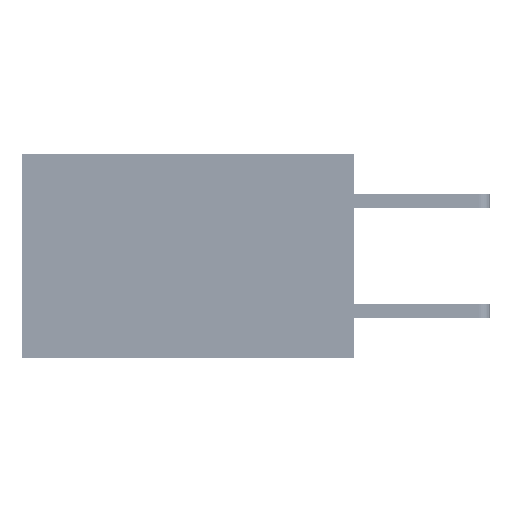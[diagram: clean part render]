
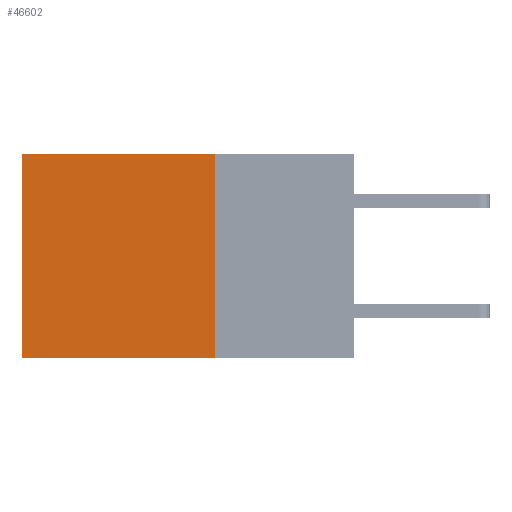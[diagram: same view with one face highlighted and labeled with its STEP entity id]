
A CAD part, left-side view. The second image highlights one B-rep face of the part: STEP entity #46602.
In plain terms, the highlighted planar face has unit normal (-1, 0, 0).
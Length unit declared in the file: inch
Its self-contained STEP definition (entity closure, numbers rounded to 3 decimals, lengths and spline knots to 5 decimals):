
#493 = VERTEX_POINT ( 'NONE', #17430 ) ;
#2474 = EDGE_CURVE ( 'NONE', #16508, #493, #9214, .T. ) ;
#2697 = EDGE_CURVE ( 'NONE', #493, #24731, #45174, .T. ) ;
#6767 = DIRECTION ( 'NONE',  ( 0., 1., 0. ) ) ;
#7314 = VERTEX_POINT ( 'NONE', #22555 ) ;
#7531 = LINE ( 'NONE', #25855, #24650 ) ;
#9214 = LINE ( 'NONE', #24003, #32315 ) ;
#10503 = CARTESIAN_POINT ( 'NONE',  ( 0.2875, 0.25, 0. ) ) ;
#10666 = PLANE ( 'NONE',  #19569 ) ;
#11275 = DIRECTION ( 'NONE',  ( 0., 1., 0. ) ) ;
#12740 = CARTESIAN_POINT ( 'NONE',  ( 0.2875, 0.25, 0. ) ) ;
#13717 = LINE ( 'NONE', #43573, #48816 ) ;
#15975 = ORIENTED_EDGE ( 'NONE', *, *, #18605, .T. ) ;
#16197 = EDGE_CURVE ( 'NONE', #16508, #7314, #7531, .T. ) ;
#16508 = VERTEX_POINT ( 'NONE', #12740 ) ;
#17430 = CARTESIAN_POINT ( 'NONE',  ( 0.2875, 0.25, -0.37 ) ) ;
#18501 = CARTESIAN_POINT ( 'NONE',  ( 0.2875, 0.25, -0.37 ) ) ;
#18605 = EDGE_CURVE ( 'NONE', #7314, #24731, #13717, .T. ) ;
#19569 = AXIS2_PLACEMENT_3D ( 'NONE', #10503, #37025, #29389 ) ;
#19674 = ORIENTED_EDGE ( 'NONE', *, *, #16197, .T. ) ;
#22555 = CARTESIAN_POINT ( 'NONE',  ( 0.2875, 0.6, 0. ) ) ;
#24003 = CARTESIAN_POINT ( 'NONE',  ( 0.2875, 0.25, 0. ) ) ;
#24650 = VECTOR ( 'NONE', #11275, 39.37008 ) ;
#24731 = VERTEX_POINT ( 'NONE', #42796 ) ;
#25855 = CARTESIAN_POINT ( 'NONE',  ( 0.2875, 0.25, 0. ) ) ;
#27207 = DIRECTION ( 'NONE',  ( 0., 0., -1. ) ) ;
#29389 = DIRECTION ( 'NONE',  ( 0., 0., -1. ) ) ;
#32315 = VECTOR ( 'NONE', #27207, 39.37008 ) ;
#37025 = DIRECTION ( 'NONE',  ( 1., 0., 0. ) ) ;
#37206 = ORIENTED_EDGE ( 'NONE', *, *, #2697, .F. ) ;
#37350 = FACE_OUTER_BOUND ( 'NONE', #39939, .T. ) ;
#39799 = VECTOR ( 'NONE', #6767, 39.37008 ) ;
#39939 = EDGE_LOOP ( 'NONE', ( #15975, #37206, #40849, #19674 ) ) ;
#40849 = ORIENTED_EDGE ( 'NONE', *, *, #2474, .F. ) ;
#42796 = CARTESIAN_POINT ( 'NONE',  ( 0.2875, 0.6, -0.37 ) ) ;
#43418 = DIRECTION ( 'NONE',  ( 0., 0., -1. ) ) ;
#43573 = CARTESIAN_POINT ( 'NONE',  ( 0.2875, 0.6, 0. ) ) ;
#45174 = LINE ( 'NONE', #18501, #39799 ) ;
#46602 = ADVANCED_FACE ( 'NONE', ( #37350 ), #10666, .F. ) ;
#48816 = VECTOR ( 'NONE', #43418, 39.37008 ) ;
